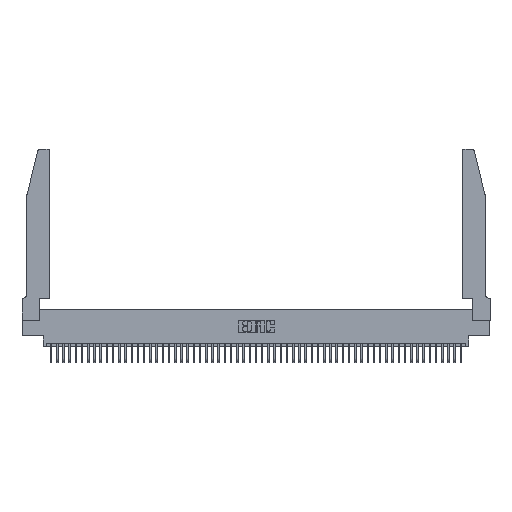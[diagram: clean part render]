
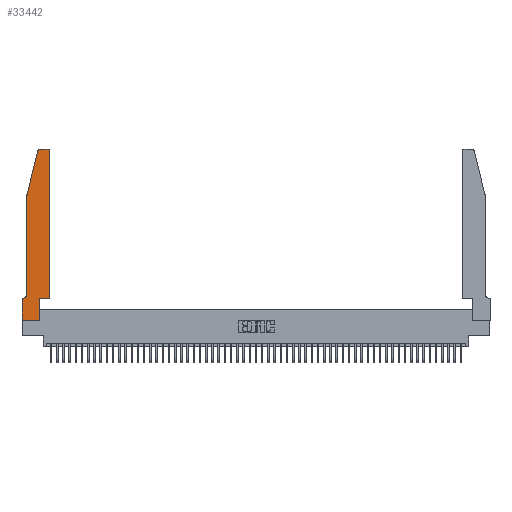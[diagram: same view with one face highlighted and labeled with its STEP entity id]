
A CAD part, top view. The second image highlights one B-rep face of the part: STEP entity #33442.
In plain terms, the highlighted planar face has unit normal (0, 0, 1).
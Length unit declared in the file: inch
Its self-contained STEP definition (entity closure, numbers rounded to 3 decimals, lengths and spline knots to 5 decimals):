
#268 = EDGE_CURVE ( 'NONE', #36642, #37983, #38156, .T. ) ;
#287 = EDGE_CURVE ( 'NONE', #49327, #36642, #27486, .T. ) ;
#808 = CARTESIAN_POINT ( 'NONE',  ( 0.284, 2.72, 0.37 ) ) ;
#1296 = LINE ( 'NONE', #8280, #32136 ) ;
#1503 = DIRECTION ( 'NONE',  ( 0., -1., 0. ) ) ;
#3107 = ORIENTED_EDGE ( 'NONE', *, *, #268, .T. ) ;
#4102 = VERTEX_POINT ( 'NONE', #23683 ) ;
#4412 = CARTESIAN_POINT ( 'NONE',  ( 0.2865, 0.35, 0.37 ) ) ;
#4453 = ORIENTED_EDGE ( 'NONE', *, *, #7319, .T. ) ;
#4849 = VERTEX_POINT ( 'NONE', #40494 ) ;
#4920 = DIRECTION ( 'NONE',  ( 1., 0., 0. ) ) ;
#6142 = CARTESIAN_POINT ( 'NONE',  ( 0.0755, 2., 0.37 ) ) ;
#6170 = VECTOR ( 'NONE', #1503, 39.37008 ) ;
#6374 = CARTESIAN_POINT ( 'NONE',  ( 0.2865, 0.35, 0.37 ) ) ;
#7319 = EDGE_CURVE ( 'NONE', #49185, #8896, #18573, .T. ) ;
#7957 = VERTEX_POINT ( 'NONE', #38091 ) ;
#8082 = PLANE ( 'NONE',  #16715 ) ;
#8126 = ORIENTED_EDGE ( 'NONE', *, *, #44662, .T. ) ;
#8280 = CARTESIAN_POINT ( 'NONE',  ( 0.2605, 2.75, 0.37 ) ) ;
#8304 = VECTOR ( 'NONE', #38212, 39.37008 ) ;
#8896 = VERTEX_POINT ( 'NONE', #32069 ) ;
#11296 = ORIENTED_EDGE ( 'NONE', *, *, #44839, .T. ) ;
#12275 = DIRECTION ( 'NONE',  ( -1., 0., 0. ) ) ;
#12504 = CARTESIAN_POINT ( 'NONE',  ( 0., 0., 0.37 ) ) ;
#13190 = ORIENTED_EDGE ( 'NONE', *, *, #37743, .T. ) ;
#13600 = DIRECTION ( 'NONE',  ( 0., 0., -1. ) ) ;
#13695 = CARTESIAN_POINT ( 'NONE',  ( 0.0755, 0.42, 0.37 ) ) ;
#14201 = CARTESIAN_POINT ( 'NONE',  ( 0.0055, 0.35, 0.37 ) ) ;
#15142 = VERTEX_POINT ( 'NONE', #47311 ) ;
#15360 = CARTESIAN_POINT ( 'NONE',  ( 0.4505, 0.35, 0.37 ) ) ;
#16081 = CARTESIAN_POINT ( 'NONE',  ( 0., 0.35, 0.37 ) ) ;
#16336 = EDGE_CURVE ( 'NONE', #25254, #38306, #43906, .T. ) ;
#16498 = DIRECTION ( 'NONE',  ( 1., 0., 0. ) ) ;
#16715 = AXIS2_PLACEMENT_3D ( 'NONE', #16081, #44180, #20123 ) ;
#17110 = DIRECTION ( 'NONE',  ( -1., 0., 0. ) ) ;
#17279 = CARTESIAN_POINT ( 'NONE',  ( 0.0755, 0.35, 0.37 ) ) ;
#17448 = ORIENTED_EDGE ( 'NONE', *, *, #45564, .T. ) ;
#17593 = VECTOR ( 'NONE', #16498, 39.37008 ) ;
#17731 = CARTESIAN_POINT ( 'NONE',  ( 0.4505, 0.35, 0.37 ) ) ;
#17808 = CARTESIAN_POINT ( 'NONE',  ( 0., 0., 0.37 ) ) ;
#18573 = LINE ( 'NONE', #17731, #39968 ) ;
#18767 = VECTOR ( 'NONE', #34005, 39.37008 ) ;
#20042 = LINE ( 'NONE', #17808, #18767 ) ;
#20123 = DIRECTION ( 'NONE',  ( 1., 0., 0. ) ) ;
#20696 = ORIENTED_EDGE ( 'NONE', *, *, #16336, .T. ) ;
#21057 = DIRECTION ( 'NONE',  ( 0., 0., 1. ) ) ;
#21722 = EDGE_CURVE ( 'NONE', #37983, #15142, #48104, .T. ) ;
#23683 = CARTESIAN_POINT ( 'NONE',  ( 0.4205, 2.75, 0.37 ) ) ;
#25224 = AXIS2_PLACEMENT_3D ( 'NONE', #45103, #21057, #49128 ) ;
#25254 = VERTEX_POINT ( 'NONE', #44747 ) ;
#27486 = LINE ( 'NONE', #29605, #6170 ) ;
#28232 = AXIS2_PLACEMENT_3D ( 'NONE', #808, #28918, #4920 ) ;
#28344 = LINE ( 'NONE', #12504, #17593 ) ;
#28623 = CARTESIAN_POINT ( 'NONE',  ( 0.284, 2.75, 0.37 ) ) ;
#28627 = EDGE_CURVE ( 'NONE', #4849, #25254, #28344, .T. ) ;
#28918 = DIRECTION ( 'NONE',  ( 0., 0., 1. ) ) ;
#28959 = VECTOR ( 'NONE', #31557, 39.37008 ) ;
#29465 = EDGE_CURVE ( 'NONE', #15142, #4849, #20042, .T. ) ;
#29605 = CARTESIAN_POINT ( 'NONE',  ( 0.0755, 2., 0.37 ) ) ;
#30378 = DIRECTION ( 'NONE',  ( 0., 1., 0. ) ) ;
#31136 = CIRCLE ( 'NONE', #25224, 0.03 ) ;
#31557 = DIRECTION ( 'NONE',  ( 1., 0., 0. ) ) ;
#32015 = VECTOR ( 'NONE', #30378, 39.37008 ) ;
#32069 = CARTESIAN_POINT ( 'NONE',  ( 0.4505, 2.72, 0.37 ) ) ;
#32136 = VECTOR ( 'NONE', #12275, 39.37008 ) ;
#33013 = EDGE_LOOP ( 'NONE', ( #33817, #17448, #8126, #39491, #3107, #45767, #49537, #37049, #20696, #11296, #4453, #13190 ) ) ;
#33442 = ADVANCED_FACE ( 'NONE', ( #40384 ), #8082, .T. ) ;
#33817 = ORIENTED_EDGE ( 'NONE', *, *, #35360, .T. ) ;
#34005 = DIRECTION ( 'NONE',  ( 0., -1., 0. ) ) ;
#35152 = CIRCLE ( 'NONE', #28232, 0.03 ) ;
#35360 = EDGE_CURVE ( 'NONE', #4102, #50722, #1296, .T. ) ;
#36202 = VECTOR ( 'NONE', #17110, 39.37008 ) ;
#36642 = VERTEX_POINT ( 'NONE', #13695 ) ;
#37049 = ORIENTED_EDGE ( 'NONE', *, *, #28627, .T. ) ;
#37682 = CARTESIAN_POINT ( 'NONE',  ( 0.0055, 0.42, 0.37 ) ) ;
#37743 = EDGE_CURVE ( 'NONE', #8896, #4102, #31136, .T. ) ;
#37796 = DIRECTION ( 'NONE',  ( 0., 1., 0. ) ) ;
#37983 = VERTEX_POINT ( 'NONE', #14201 ) ;
#38091 = CARTESIAN_POINT ( 'NONE',  ( 0.25487, 2.72718, 0.37 ) ) ;
#38156 = CIRCLE ( 'NONE', #44372, 0.07 ) ;
#38212 = DIRECTION ( 'NONE',  ( -0.239, -0.971, 0. ) ) ;
#38306 = VERTEX_POINT ( 'NONE', #4412 ) ;
#39008 = LINE ( 'NONE', #6142, #8304 ) ;
#39491 = ORIENTED_EDGE ( 'NONE', *, *, #287, .T. ) ;
#39968 = VECTOR ( 'NONE', #37796, 39.37008 ) ;
#40384 = FACE_OUTER_BOUND ( 'NONE', #33013, .T. ) ;
#40494 = CARTESIAN_POINT ( 'NONE',  ( 0., 0., 0.37 ) ) ;
#41672 = DIRECTION ( 'NONE',  ( -1., 0., 0. ) ) ;
#43632 = CARTESIAN_POINT ( 'NONE',  ( 0.0755, 2., 0.37 ) ) ;
#43906 = LINE ( 'NONE', #6374, #32015 ) ;
#44180 = DIRECTION ( 'NONE',  ( 0., 0., 1. ) ) ;
#44372 = AXIS2_PLACEMENT_3D ( 'NONE', #37682, #13600, #41672 ) ;
#44662 = EDGE_CURVE ( 'NONE', #7957, #49327, #39008, .T. ) ;
#44747 = CARTESIAN_POINT ( 'NONE',  ( 0.2865, 0., 0.37 ) ) ;
#44839 = EDGE_CURVE ( 'NONE', #38306, #49185, #50289, .T. ) ;
#45103 = CARTESIAN_POINT ( 'NONE',  ( 0.4205, 2.72, 0.37 ) ) ;
#45564 = EDGE_CURVE ( 'NONE', #50722, #7957, #35152, .T. ) ;
#45767 = ORIENTED_EDGE ( 'NONE', *, *, #21722, .T. ) ;
#47311 = CARTESIAN_POINT ( 'NONE',  ( 0., 0.35, 0.37 ) ) ;
#48104 = LINE ( 'NONE', #17279, #36202 ) ;
#49128 = DIRECTION ( 'NONE',  ( 1., 0., 0. ) ) ;
#49185 = VERTEX_POINT ( 'NONE', #50491 ) ;
#49327 = VERTEX_POINT ( 'NONE', #43632 ) ;
#49537 = ORIENTED_EDGE ( 'NONE', *, *, #29465, .T. ) ;
#50289 = LINE ( 'NONE', #15360, #28959 ) ;
#50491 = CARTESIAN_POINT ( 'NONE',  ( 0.4505, 0.35, 0.37 ) ) ;
#50722 = VERTEX_POINT ( 'NONE', #28623 ) ;
